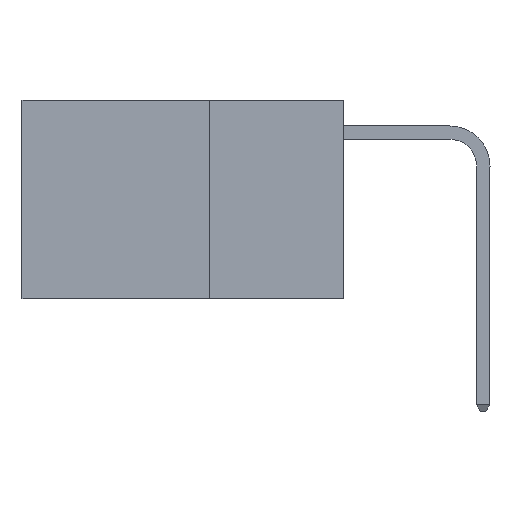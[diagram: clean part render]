
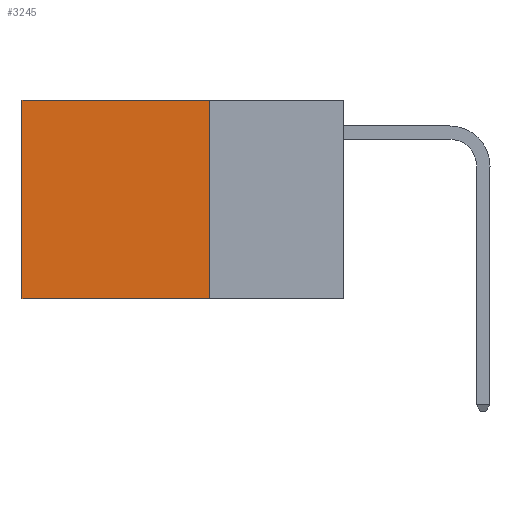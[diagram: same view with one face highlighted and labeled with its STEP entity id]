
A CAD part, left-side view. The second image highlights one B-rep face of the part: STEP entity #3245.
In plain terms, the highlighted planar face has unit normal (-1, 0, 0).
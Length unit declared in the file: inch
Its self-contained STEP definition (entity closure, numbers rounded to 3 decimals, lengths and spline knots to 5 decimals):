
#8 = ORIENTED_EDGE ( 'NONE', *, *, #9031, .T. ) ;
#65 = DIRECTION ( 'NONE',  ( 0., 0., -1. ) ) ;
#125 = VECTOR ( 'NONE', #3521, 39.37008 ) ;
#668 = CARTESIAN_POINT ( 'NONE',  ( 0.2625, 0.25, -0.37 ) ) ;
#876 = CARTESIAN_POINT ( 'NONE',  ( 0.2625, 0.25, 0. ) ) ;
#950 = CARTESIAN_POINT ( 'NONE',  ( 0.2625, 0.6, 0. ) ) ;
#1470 = EDGE_LOOP ( 'NONE', ( #3144, #3048, #5767, #8 ) ) ;
#1868 = CARTESIAN_POINT ( 'NONE',  ( 0.2625, 0.25, 0. ) ) ;
#1948 = EDGE_CURVE ( 'NONE', #7655, #2136, #2202, .T. ) ;
#2031 = DIRECTION ( 'NONE',  ( 0., 1., 0. ) ) ;
#2095 = AXIS2_PLACEMENT_3D ( 'NONE', #8539, #3749, #9323 ) ;
#2136 = VERTEX_POINT ( 'NONE', #5792 ) ;
#2202 = LINE ( 'NONE', #2929, #6391 ) ;
#2418 = LINE ( 'NONE', #876, #125 ) ;
#2641 = LINE ( 'NONE', #8624, #4636 ) ;
#2830 = EDGE_CURVE ( 'NONE', #3874, #7655, #2641, .T. ) ;
#2929 = CARTESIAN_POINT ( 'NONE',  ( 0.2625, 0.25, -0.37 ) ) ;
#3048 = ORIENTED_EDGE ( 'NONE', *, *, #1948, .F. ) ;
#3144 = ORIENTED_EDGE ( 'NONE', *, *, #7854, .T. ) ;
#3245 = ADVANCED_FACE ( 'NONE', ( #8701 ), #7758, .F. ) ;
#3521 = DIRECTION ( 'NONE',  ( 0., 1., 0. ) ) ;
#3749 = DIRECTION ( 'NONE',  ( 1., 0., 0. ) ) ;
#3874 = VERTEX_POINT ( 'NONE', #1868 ) ;
#4545 = CARTESIAN_POINT ( 'NONE',  ( 0.2625, 0.6, 0. ) ) ;
#4636 = VECTOR ( 'NONE', #7838, 39.37008 ) ;
#4808 = VECTOR ( 'NONE', #65, 39.37008 ) ;
#5767 = ORIENTED_EDGE ( 'NONE', *, *, #2830, .F. ) ;
#5792 = CARTESIAN_POINT ( 'NONE',  ( 0.2625, 0.6, -0.37 ) ) ;
#6391 = VECTOR ( 'NONE', #2031, 39.37008 ) ;
#7655 = VERTEX_POINT ( 'NONE', #668 ) ;
#7758 = PLANE ( 'NONE',  #2095 ) ;
#7838 = DIRECTION ( 'NONE',  ( 0., 0., -1. ) ) ;
#7854 = EDGE_CURVE ( 'NONE', #9999, #2136, #9004, .T. ) ;
#8539 = CARTESIAN_POINT ( 'NONE',  ( 0.2625, 0.25, 0. ) ) ;
#8624 = CARTESIAN_POINT ( 'NONE',  ( 0.2625, 0.25, 0. ) ) ;
#8701 = FACE_OUTER_BOUND ( 'NONE', #1470, .T. ) ;
#9004 = LINE ( 'NONE', #950, #4808 ) ;
#9031 = EDGE_CURVE ( 'NONE', #3874, #9999, #2418, .T. ) ;
#9323 = DIRECTION ( 'NONE',  ( 0., 0., -1. ) ) ;
#9999 = VERTEX_POINT ( 'NONE', #4545 ) ;
